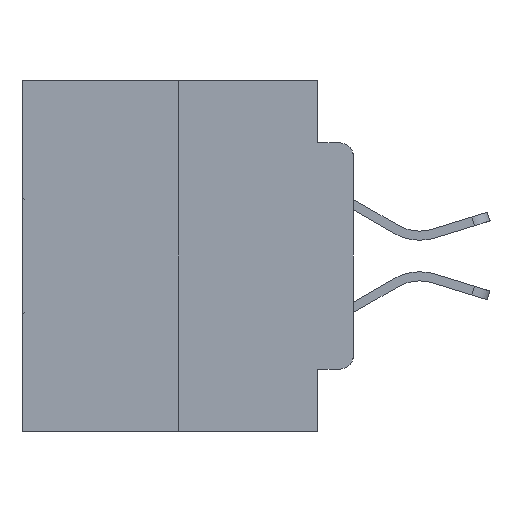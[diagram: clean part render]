
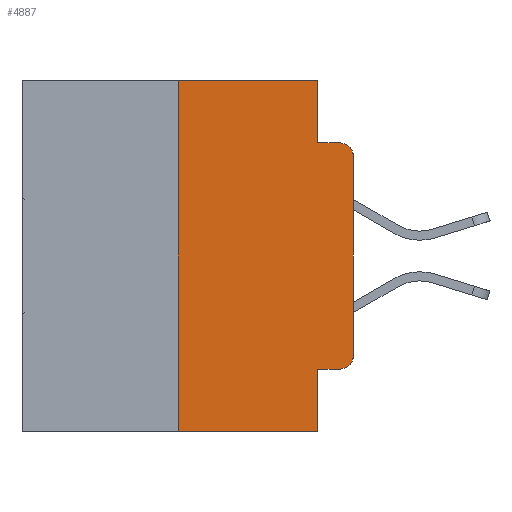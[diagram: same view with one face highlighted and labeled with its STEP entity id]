
A CAD part, left-side view. The second image highlights one B-rep face of the part: STEP entity #4887.
In plain terms, the highlighted planar face has unit normal (-1, 0, 0).
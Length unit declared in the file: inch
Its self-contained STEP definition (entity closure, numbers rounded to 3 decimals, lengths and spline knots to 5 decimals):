
#321 = DIRECTION ( 'NONE',  ( 0., 0., 1. ) ) ;
#590 = CARTESIAN_POINT ( 'NONE',  ( 0., 0.25, -0.5 ) ) ;
#1646 = VECTOR ( 'NONE', #7835, 39.37008 ) ;
#1693 = VERTEX_POINT ( 'NONE', #590 ) ;
#1908 = CARTESIAN_POINT ( 'NONE',  ( 0., 0., 0. ) ) ;
#2337 = PLANE ( 'NONE',  #10185 ) ;
#2731 = ORIENTED_EDGE ( 'NONE', *, *, #13111, .F. ) ;
#2744 = EDGE_CURVE ( 'NONE', #1693, #25542, #19748, .T. ) ;
#3006 = CARTESIAN_POINT ( 'NONE',  ( 0., 0.473, 0. ) ) ;
#3009 = EDGE_CURVE ( 'NONE', #8526, #25542, #7712, .T. ) ;
#3216 = CARTESIAN_POINT ( 'NONE',  ( 0., 0., -0.3915 ) ) ;
#3219 = VECTOR ( 'NONE', #26613, 39.37008 ) ;
#3392 = ORIENTED_EDGE ( 'NONE', *, *, #13661, .T. ) ;
#3400 = VERTEX_POINT ( 'NONE', #3770 ) ;
#3477 = VERTEX_POINT ( 'NONE', #12124 ) ;
#3766 = EDGE_CURVE ( 'NONE', #27658, #27383, #22706, .T. ) ;
#3770 = CARTESIAN_POINT ( 'NONE',  ( 0., 0.051, 0. ) ) ;
#3996 = CARTESIAN_POINT ( 'NONE',  ( 0., 0.051, 0. ) ) ;
#4887 = ADVANCED_FACE ( 'NONE', ( #5492 ), #2337, .F. ) ;
#5211 = VECTOR ( 'NONE', #321, 39.37008 ) ;
#5492 = FACE_OUTER_BOUND ( 'NONE', #20715, .T. ) ;
#5880 = VECTOR ( 'NONE', #24840, 39.37008 ) ;
#5969 = DIRECTION ( 'NONE',  ( -1., 0., 0. ) ) ;
#6080 = DIRECTION ( 'NONE',  ( 0., -1., 0. ) ) ;
#6246 = EDGE_CURVE ( 'NONE', #1693, #19121, #6828, .T. ) ;
#6457 = CARTESIAN_POINT ( 'NONE',  ( 0., 0.02, -0.0885 ) ) ;
#6828 = LINE ( 'NONE', #20423, #22908 ) ;
#7712 = LINE ( 'NONE', #3996, #1646 ) ;
#7835 = DIRECTION ( 'NONE',  ( 0., 0., -1. ) ) ;
#8488 = CARTESIAN_POINT ( 'NONE',  ( 0., 0.051, -0.0885 ) ) ;
#8526 = VERTEX_POINT ( 'NONE', #24424 ) ;
#8697 = CARTESIAN_POINT ( 'NONE',  ( 0., 0.02, -0.3915 ) ) ;
#9182 = LINE ( 'NONE', #13611, #3219 ) ;
#9678 = LINE ( 'NONE', #10547, #20659 ) ;
#10050 = ORIENTED_EDGE ( 'NONE', *, *, #3766, .T. ) ;
#10185 = AXIS2_PLACEMENT_3D ( 'NONE', #3006, #14135, #17193 ) ;
#10371 = CIRCLE ( 'NONE', #16466, 0.02 ) ;
#10547 = CARTESIAN_POINT ( 'NONE',  ( 0., 0.473, 0. ) ) ;
#10715 = DIRECTION ( 'NONE',  ( 0., -1., 0. ) ) ;
#10923 = DIRECTION ( 'NONE',  ( 0., 0., -1. ) ) ;
#11155 = VECTOR ( 'NONE', #10715, 39.37008 ) ;
#12124 = CARTESIAN_POINT ( 'NONE',  ( 0., 0.02, -0.4115 ) ) ;
#12474 = LINE ( 'NONE', #16250, #5880 ) ;
#13111 = EDGE_CURVE ( 'NONE', #3400, #14172, #12474, .T. ) ;
#13222 = ORIENTED_EDGE ( 'NONE', *, *, #2744, .T. ) ;
#13611 = CARTESIAN_POINT ( 'NONE',  ( 0., 0.051, -0.4115 ) ) ;
#13661 = EDGE_CURVE ( 'NONE', #27383, #13806, #10371, .T. ) ;
#13806 = VERTEX_POINT ( 'NONE', #6457 ) ;
#14135 = DIRECTION ( 'NONE',  ( 1., 0., 0. ) ) ;
#14172 = VERTEX_POINT ( 'NONE', #22912 ) ;
#14641 = VECTOR ( 'NONE', #18500, 39.37008 ) ;
#15614 = CARTESIAN_POINT ( 'NONE',  ( 0., 0., -0.1085 ) ) ;
#15694 = ORIENTED_EDGE ( 'NONE', *, *, #17361, .T. ) ;
#15973 = ORIENTED_EDGE ( 'NONE', *, *, #18978, .F. ) ;
#16237 = CIRCLE ( 'NONE', #20888, 0.02 ) ;
#16250 = CARTESIAN_POINT ( 'NONE',  ( 0., 0.051, 0. ) ) ;
#16330 = ORIENTED_EDGE ( 'NONE', *, *, #28206, .T. ) ;
#16466 = AXIS2_PLACEMENT_3D ( 'NONE', #19183, #5969, #21343 ) ;
#17193 = DIRECTION ( 'NONE',  ( 0., 0., -1. ) ) ;
#17361 = EDGE_CURVE ( 'NONE', #8526, #3477, #9182, .T. ) ;
#17972 = ORIENTED_EDGE ( 'NONE', *, *, #3009, .F. ) ;
#18500 = DIRECTION ( 'NONE',  ( 0., -1., 0. ) ) ;
#18978 = EDGE_CURVE ( 'NONE', #14172, #13806, #28486, .T. ) ;
#19121 = VERTEX_POINT ( 'NONE', #28479 ) ;
#19183 = CARTESIAN_POINT ( 'NONE',  ( 0., 0.02, -0.1085 ) ) ;
#19587 = CARTESIAN_POINT ( 'NONE',  ( 0., 0.051, -0.5 ) ) ;
#19748 = LINE ( 'NONE', #22255, #14641 ) ;
#20423 = CARTESIAN_POINT ( 'NONE',  ( 0., 0.25, 0. ) ) ;
#20659 = VECTOR ( 'NONE', #6080, 39.37008 ) ;
#20715 = EDGE_LOOP ( 'NONE', ( #10050, #3392, #15973, #2731, #24032, #22009, #13222, #17972, #15694, #16330 ) ) ;
#20888 = AXIS2_PLACEMENT_3D ( 'NONE', #8697, #23971, #10923 ) ;
#21343 = DIRECTION ( 'NONE',  ( 0., 0., -1. ) ) ;
#22009 = ORIENTED_EDGE ( 'NONE', *, *, #6246, .F. ) ;
#22255 = CARTESIAN_POINT ( 'NONE',  ( 0., 0.473, -0.5 ) ) ;
#22706 = LINE ( 'NONE', #1908, #5211 ) ;
#22908 = VECTOR ( 'NONE', #24762, 39.37008 ) ;
#22912 = CARTESIAN_POINT ( 'NONE',  ( 0., 0.051, -0.0885 ) ) ;
#23971 = DIRECTION ( 'NONE',  ( -1., 0., 0. ) ) ;
#24032 = ORIENTED_EDGE ( 'NONE', *, *, #27836, .F. ) ;
#24424 = CARTESIAN_POINT ( 'NONE',  ( 0., 0.051, -0.4115 ) ) ;
#24762 = DIRECTION ( 'NONE',  ( 0., 0., 1. ) ) ;
#24840 = DIRECTION ( 'NONE',  ( 0., 0., -1. ) ) ;
#25542 = VERTEX_POINT ( 'NONE', #19587 ) ;
#26613 = DIRECTION ( 'NONE',  ( 0., -1., 0. ) ) ;
#27383 = VERTEX_POINT ( 'NONE', #15614 ) ;
#27658 = VERTEX_POINT ( 'NONE', #3216 ) ;
#27836 = EDGE_CURVE ( 'NONE', #19121, #3400, #9678, .T. ) ;
#28206 = EDGE_CURVE ( 'NONE', #3477, #27658, #16237, .T. ) ;
#28479 = CARTESIAN_POINT ( 'NONE',  ( 0., 0.25, 0. ) ) ;
#28486 = LINE ( 'NONE', #8488, #11155 ) ;
